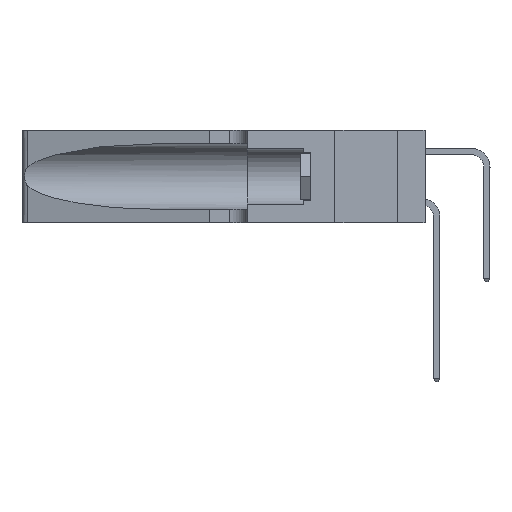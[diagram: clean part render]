
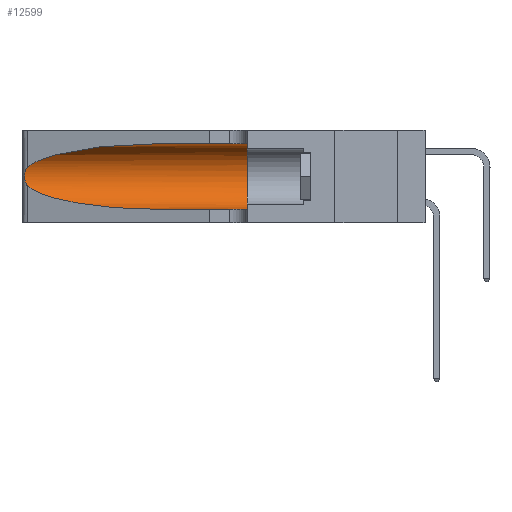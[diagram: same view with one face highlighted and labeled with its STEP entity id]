
A CAD part, left-side view. The second image highlights one B-rep face of the part: STEP entity #12599.
In plain terms, the highlighted cylindrical face has radius 3.308 mm (diameter 6.617 mm), a partial arc.
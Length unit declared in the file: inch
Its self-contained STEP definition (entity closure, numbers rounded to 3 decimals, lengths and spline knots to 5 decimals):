
#509 = CARTESIAN_POINT ( 'NONE',  ( 0.25789, 1.23486, 0.15765 ) ) ;
#723 = CARTESIAN_POINT ( 'NONE',  ( 0.1305, 1.61858, 0.31525 ) ) ;
#1322 = DIRECTION ( 'NONE',  ( 0., 0., -1. ) ) ;
#2526 = B_SPLINE_CURVE_WITH_KNOTS ( 'NONE', 3,
 ( #19836, #14342, #25319, #8907, #28048, #11715, #30762, #14453, #33477, #17209, #509, #19961, #3374, #22693 ),
 .UNSPECIFIED., .F., .F.,
 ( 4, 2, 2, 2, 2, 2, 4 ),
 ( 0., 0.00027, 0.00053, 0.00107, 0.0016, 0.00187, 0.00214 ),
 .UNSPECIFIED. ) ;
#2943 = CARTESIAN_POINT ( 'NONE',  ( 0.1305, 0.72297, 0.31525 ) ) ;
#3374 = CARTESIAN_POINT ( 'NONE',  ( 0.25555, 1.22993, 0.14849 ) ) ;
#3658 =( BOUNDED_CURVE ( )  B_SPLINE_CURVE ( 3, ( #28192, #19996, #14604, #33623 ),
 .UNSPECIFIED., .F., .T. ) 
 B_SPLINE_CURVE_WITH_KNOTS ( ( 4, 4 ),
 ( 1.5708, 2.84003 ),
 .UNSPECIFIED. ) 
 CURVE ( )  GEOMETRIC_REPRESENTATION_ITEM ( )  RATIONAL_B_SPLINE_CURVE ( ( 1., 0.87, 0.87, 1. ) ) 
 REPRESENTATION_ITEM ( '' )  );
#3971 = CARTESIAN_POINT ( 'NONE',  ( 0.1305, 1.61858, 0.05475 ) ) ;
#4056 = DIRECTION ( 'NONE',  ( 0., -1., 0. ) ) ;
#4647 = EDGE_CURVE ( 'NONE', #31170, #20348, #21460, .T. ) ;
#5498 = ORIENTED_EDGE ( 'NONE', *, *, #21806, .T. ) ;
#6276 = VERTEX_POINT ( 'NONE', #32300 ) ;
#6340 = LINE ( 'NONE', #723, #24787 ) ;
#6420 =( BOUNDED_CURVE ( )  B_SPLINE_CURVE ( 3, ( #23753, #21140, #12980, #32045 ),
 .UNSPECIFIED., .F., .F. ) 
 B_SPLINE_CURVE_WITH_KNOTS ( ( 4, 4 ),
 ( 3.44316, 4.71239 ),
 .UNSPECIFIED. ) 
 CURVE ( )  GEOMETRIC_REPRESENTATION_ITEM ( )  RATIONAL_B_SPLINE_CURVE ( ( 1., 0.87, 0.87, 1. ) ) 
 REPRESENTATION_ITEM ( '' )  );
#6604 = EDGE_CURVE ( 'NONE', #10469, #34587, #6340, .T. ) ;
#6828 = DIRECTION ( 'NONE',  ( 0., -1., 0. ) ) ;
#7510 = EDGE_LOOP ( 'NONE', ( #33959, #16217, #5498, #26495, #23594, #31899 ) ) ;
#8907 = CARTESIAN_POINT ( 'NONE',  ( 0.25787, 1.23484, 0.2124 ) ) ;
#10469 = VERTEX_POINT ( 'NONE', #2943 ) ;
#11715 = CARTESIAN_POINT ( 'NONE',  ( 0.26018, 1.23835, 0.19895 ) ) ;
#12429 = CIRCLE ( 'NONE', #25908, 0.13025 ) ;
#12599 = ADVANCED_FACE ( 'NONE', ( #29046 ), #35376, .F. ) ;
#12943 = VERTEX_POINT ( 'NONE', #18802 ) ;
#12980 = CARTESIAN_POINT ( 'NONE',  ( 0.18966, 0.96281, 0.05475 ) ) ;
#14342 = CARTESIAN_POINT ( 'NONE',  ( 0.25555, 1.22994, 0.2215 ) ) ;
#14453 = CARTESIAN_POINT ( 'NONE',  ( 0.26075, 1.23896, 0.178 ) ) ;
#14604 = CARTESIAN_POINT ( 'NONE',  ( 0.2373, 1.15595, 0.28018 ) ) ;
#15749 = EDGE_CURVE ( 'NONE', #6276, #12943, #2526, .T. ) ;
#16140 = DIRECTION ( 'NONE',  ( 0., 1., 0. ) ) ;
#16217 = ORIENTED_EDGE ( 'NONE', *, *, #15749, .T. ) ;
#17209 = CARTESIAN_POINT ( 'NONE',  ( 0.25856, 1.23593, 0.16098 ) ) ;
#17969 = CARTESIAN_POINT ( 'NONE',  ( 0.1305, 1.61858, 0.185 ) ) ;
#18802 = CARTESIAN_POINT ( 'NONE',  ( 0.25487, 1.22718, 0.14631 ) ) ;
#19836 = CARTESIAN_POINT ( 'NONE',  ( 0.25487, 1.22718, 0.22369 ) ) ;
#19961 = CARTESIAN_POINT ( 'NONE',  ( 0.25639, 1.23186, 0.15144 ) ) ;
#19996 = CARTESIAN_POINT ( 'NONE',  ( 0.18966, 0.96281, 0.31525 ) ) ;
#20348 = VERTEX_POINT ( 'NONE', #23376 ) ;
#21140 = CARTESIAN_POINT ( 'NONE',  ( 0.2373, 1.15595, 0.08982 ) ) ;
#21460 = LINE ( 'NONE', #3971, #34170 ) ;
#21806 = EDGE_CURVE ( 'NONE', #12943, #31170, #6420, .T. ) ;
#22693 = CARTESIAN_POINT ( 'NONE',  ( 0.25487, 1.22718, 0.14631 ) ) ;
#23376 = CARTESIAN_POINT ( 'NONE',  ( 0.1305, 0.35, 0.05475 ) ) ;
#23512 = EDGE_CURVE ( 'NONE', #34587, #20348, #12429, .T. ) ;
#23594 = ORIENTED_EDGE ( 'NONE', *, *, #23512, .F. ) ;
#23753 = CARTESIAN_POINT ( 'NONE',  ( 0.25487, 1.22718, 0.14631 ) ) ;
#24787 = VECTOR ( 'NONE', #30965, 39.37008 ) ;
#24850 = CARTESIAN_POINT ( 'NONE',  ( 0.1305, 0.72297, 0.05475 ) ) ;
#25319 = CARTESIAN_POINT ( 'NONE',  ( 0.25639, 1.23184, 0.21858 ) ) ;
#25908 = AXIS2_PLACEMENT_3D ( 'NONE', #32426, #16140, #35135 ) ;
#26495 = ORIENTED_EDGE ( 'NONE', *, *, #4647, .T. ) ;
#27227 = AXIS2_PLACEMENT_3D ( 'NONE', #17969, #4056, #1322 ) ;
#28048 = CARTESIAN_POINT ( 'NONE',  ( 0.25854, 1.2359, 0.20912 ) ) ;
#28077 = CARTESIAN_POINT ( 'NONE',  ( 0.1305, 0.35, 0.31525 ) ) ;
#28192 = CARTESIAN_POINT ( 'NONE',  ( 0.1305, 0.72297, 0.31525 ) ) ;
#29046 = FACE_OUTER_BOUND ( 'NONE', #7510, .T. ) ;
#30762 = CARTESIAN_POINT ( 'NONE',  ( 0.26075, 1.23896, 0.19203 ) ) ;
#30965 = DIRECTION ( 'NONE',  ( 0., -1., 0. ) ) ;
#31170 = VERTEX_POINT ( 'NONE', #24850 ) ;
#31899 = ORIENTED_EDGE ( 'NONE', *, *, #6604, .F. ) ;
#32045 = CARTESIAN_POINT ( 'NONE',  ( 0.1305, 0.72297, 0.05475 ) ) ;
#32300 = CARTESIAN_POINT ( 'NONE',  ( 0.25487, 1.22718, 0.22369 ) ) ;
#32426 = CARTESIAN_POINT ( 'NONE',  ( 0.1305, 0.35, 0.185 ) ) ;
#33477 = CARTESIAN_POINT ( 'NONE',  ( 0.26017, 1.23833, 0.17102 ) ) ;
#33623 = CARTESIAN_POINT ( 'NONE',  ( 0.25487, 1.22718, 0.22369 ) ) ;
#33959 = ORIENTED_EDGE ( 'NONE', *, *, #34614, .T. ) ;
#34170 = VECTOR ( 'NONE', #6828, 39.37008 ) ;
#34587 = VERTEX_POINT ( 'NONE', #28077 ) ;
#34614 = EDGE_CURVE ( 'NONE', #10469, #6276, #3658, .T. ) ;
#35135 = DIRECTION ( 'NONE',  ( 0., 0., 1. ) ) ;
#35376 = CYLINDRICAL_SURFACE ( 'NONE', #27227, 0.13025 ) ;
